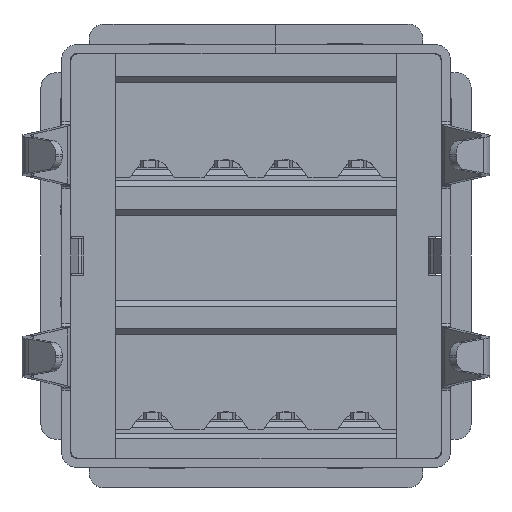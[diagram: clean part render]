
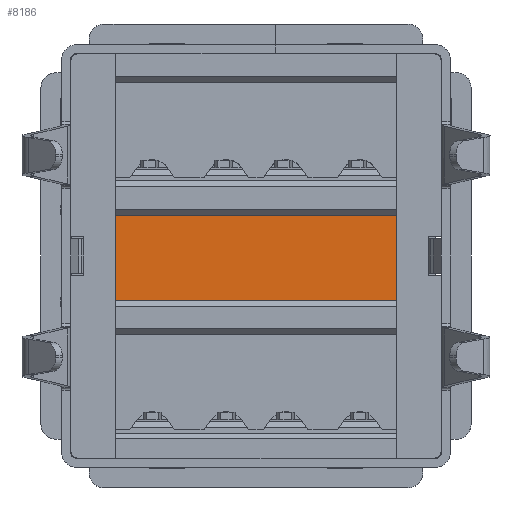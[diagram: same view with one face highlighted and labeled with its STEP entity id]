
A CAD part, front view. The second image highlights one B-rep face of the part: STEP entity #8186.
In plain terms, the highlighted face is planar.
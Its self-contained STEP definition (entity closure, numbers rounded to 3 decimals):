
#328 = ORIENTED_EDGE ( 'NONE', *, *, #25933, .F. ) ;
#919 = CARTESIAN_POINT ( 'NONE',  ( 0., -0.795, -3.62 ) ) ;
#2196 = VERTEX_POINT ( 'NONE', #41740 ) ;
#3959 = DIRECTION ( 'NONE',  ( 0., -1., 0. ) ) ;
#4483 = ORIENTED_EDGE ( 'NONE', *, *, #43528, .F. ) ;
#4570 = CARTESIAN_POINT ( 'NONE',  ( -4.75, -0.795, -3.62 ) ) ;
#4756 = VECTOR ( 'NONE', #7904, 1000. ) ;
#4891 = CARTESIAN_POINT ( 'NONE',  ( 4.75, 2.075, -3.62 ) ) ;
#4928 = DIRECTION ( 'NONE',  ( 0., -1., 0. ) ) ;
#6865 = CARTESIAN_POINT ( 'NONE',  ( 0., 2.075, -3.62 ) ) ;
#7904 = DIRECTION ( 'NONE',  ( -1., 0., 0. ) ) ;
#7969 = CARTESIAN_POINT ( 'NONE',  ( 0., 0.64, -3.62 ) ) ;
#8186 = ADVANCED_FACE ( 'NONE', ( #44244 ), #48742, .F. ) ;
#9035 = ORIENTED_EDGE ( 'NONE', *, *, #34005, .F. ) ;
#9604 = VECTOR ( 'NONE', #4928, 1000. ) ;
#11289 = EDGE_CURVE ( 'NONE', #51532, #16332, #49171, .T. ) ;
#16332 = VERTEX_POINT ( 'NONE', #35654 ) ;
#19015 = EDGE_LOOP ( 'NONE', ( #9035, #328, #34574, #4483 ) ) ;
#20563 = CARTESIAN_POINT ( 'NONE',  ( 4.75, 0.58, -3.62 ) ) ;
#23806 = LINE ( 'NONE', #919, #39758 ) ;
#23934 = AXIS2_PLACEMENT_3D ( 'NONE', #7969, #34788, #36005 ) ;
#25933 = EDGE_CURVE ( 'NONE', #51532, #2196, #35169, .T. ) ;
#31993 = DIRECTION ( 'NONE',  ( 1., 0., 0. ) ) ;
#32529 = LINE ( 'NONE', #40494, #32535 ) ;
#32535 = VECTOR ( 'NONE', #3959, 1000. ) ;
#34005 = EDGE_CURVE ( 'NONE', #2196, #50089, #32529, .T. ) ;
#34574 = ORIENTED_EDGE ( 'NONE', *, *, #11289, .T. ) ;
#34788 = DIRECTION ( 'NONE',  ( 0., 0., 1. ) ) ;
#35169 = LINE ( 'NONE', #6865, #4756 ) ;
#35654 = CARTESIAN_POINT ( 'NONE',  ( 4.75, -0.795, -3.62 ) ) ;
#36005 = DIRECTION ( 'NONE',  ( 1., 0., 0. ) ) ;
#39758 = VECTOR ( 'NONE', #31993, 1000. ) ;
#40494 = CARTESIAN_POINT ( 'NONE',  ( -4.75, 0.58, -3.62 ) ) ;
#41740 = CARTESIAN_POINT ( 'NONE',  ( -4.75, 2.075, -3.62 ) ) ;
#43528 = EDGE_CURVE ( 'NONE', #50089, #16332, #23806, .T. ) ;
#44244 = FACE_OUTER_BOUND ( 'NONE', #19015, .T. ) ;
#48742 = PLANE ( 'NONE',  #23934 ) ;
#49171 = LINE ( 'NONE', #20563, #9604 ) ;
#50089 = VERTEX_POINT ( 'NONE', #4570 ) ;
#51532 = VERTEX_POINT ( 'NONE', #4891 ) ;
